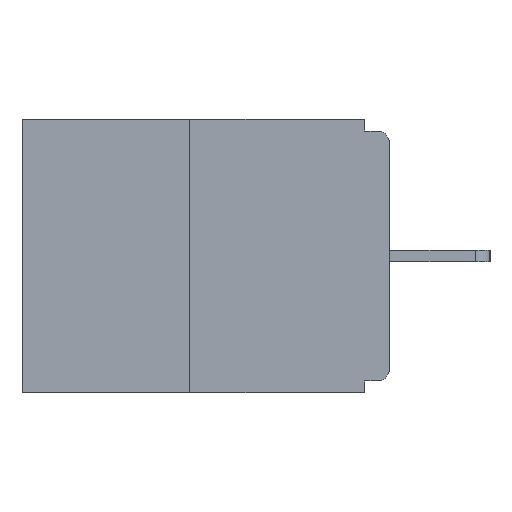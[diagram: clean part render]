
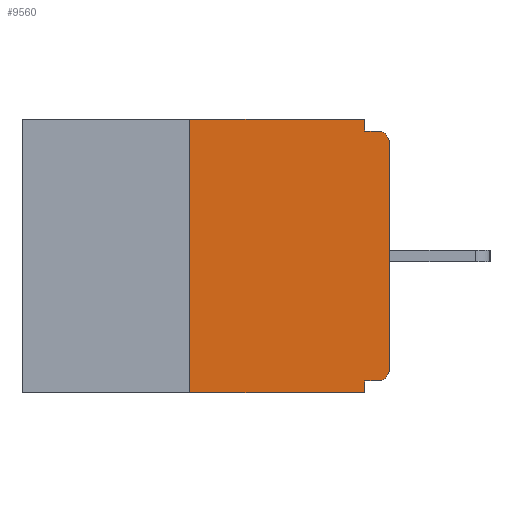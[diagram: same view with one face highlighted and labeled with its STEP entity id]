
A CAD part, left-side view. The second image highlights one B-rep face of the part: STEP entity #9560.
In plain terms, the highlighted planar face has unit normal (-1, 0, 0).
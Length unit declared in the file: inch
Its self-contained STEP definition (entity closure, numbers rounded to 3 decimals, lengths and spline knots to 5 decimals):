
#99 = DIRECTION ( 'NONE',  ( 0., 0., 1. ) ) ;
#216 = ORIENTED_EDGE ( 'NONE', *, *, #5805, .F. ) ;
#753 = CARTESIAN_POINT ( 'NONE',  ( 0., 0.015, -0.328 ) ) ;
#810 = CARTESIAN_POINT ( 'NONE',  ( 0., 0.031, -0.328 ) ) ;
#871 = CARTESIAN_POINT ( 'NONE',  ( 0., 0.031, -0.015 ) ) ;
#1136 = VERTEX_POINT ( 'NONE', #871 ) ;
#1218 = LINE ( 'NONE', #10630, #3460 ) ;
#1287 = AXIS2_PLACEMENT_3D ( 'NONE', #2479, #9513, #3595 ) ;
#1617 = CARTESIAN_POINT ( 'NONE',  ( 0., 0.25, 0. ) ) ;
#1647 = EDGE_CURVE ( 'NONE', #8354, #12426, #13458, .T. ) ;
#1669 = ORIENTED_EDGE ( 'NONE', *, *, #9038, .F. ) ;
#1750 = EDGE_CURVE ( 'NONE', #1136, #12426, #6166, .T. ) ;
#1998 = VERTEX_POINT ( 'NONE', #753 ) ;
#2083 = ORIENTED_EDGE ( 'NONE', *, *, #9638, .F. ) ;
#2479 = CARTESIAN_POINT ( 'NONE',  ( 0., 0.015, -0.313 ) ) ;
#2496 = AXIS2_PLACEMENT_3D ( 'NONE', #7346, #9879, #7579 ) ;
#2565 = VECTOR ( 'NONE', #99, 39.37008 ) ;
#2848 = EDGE_CURVE ( 'NONE', #10199, #1136, #1218, .T. ) ;
#2975 = VERTEX_POINT ( 'NONE', #11094 ) ;
#3161 = CARTESIAN_POINT ( 'NONE',  ( 0., 0.031, 0. ) ) ;
#3400 = CARTESIAN_POINT ( 'NONE',  ( 0., 0., -0.328 ) ) ;
#3460 = VECTOR ( 'NONE', #14411, 39.37008 ) ;
#3528 = DIRECTION ( 'NONE',  ( 0., -1., 0. ) ) ;
#3595 = DIRECTION ( 'NONE',  ( 0., 0., -1. ) ) ;
#4274 = VECTOR ( 'NONE', #14276, 39.37008 ) ;
#4645 = CARTESIAN_POINT ( 'NONE',  ( 0., 0., 0. ) ) ;
#4684 = DIRECTION ( 'NONE',  ( -1., 0., 0. ) ) ;
#4777 = VERTEX_POINT ( 'NONE', #6903 ) ;
#4787 = VERTEX_POINT ( 'NONE', #810 ) ;
#5148 = FACE_OUTER_BOUND ( 'NONE', #13052, .T. ) ;
#5202 = ORIENTED_EDGE ( 'NONE', *, *, #1750, .F. ) ;
#5406 = DIRECTION ( 'NONE',  ( 0., 0., -1. ) ) ;
#5527 = CARTESIAN_POINT ( 'NONE',  ( 0., 0.25, -0.343 ) ) ;
#5589 = VERTEX_POINT ( 'NONE', #5527 ) ;
#5799 = LINE ( 'NONE', #7056, #11694 ) ;
#5805 = EDGE_CURVE ( 'NONE', #1998, #4787, #15034, .T. ) ;
#6166 = LINE ( 'NONE', #10734, #4274 ) ;
#6281 = DIRECTION ( 'NONE',  ( 0., -1., 0. ) ) ;
#6903 = CARTESIAN_POINT ( 'NONE',  ( 0., 0.25, 0. ) ) ;
#7026 = CIRCLE ( 'NONE', #1287, 0.015 ) ;
#7030 = CARTESIAN_POINT ( 'NONE',  ( 0., 0.015, -0.03 ) ) ;
#7056 = CARTESIAN_POINT ( 'NONE',  ( 0., 0.46, 0. ) ) ;
#7135 = VECTOR ( 'NONE', #5406, 39.37008 ) ;
#7346 = CARTESIAN_POINT ( 'NONE',  ( 0., 0.46, 0. ) ) ;
#7377 = EDGE_CURVE ( 'NONE', #5589, #2975, #14381, .T. ) ;
#7572 = EDGE_CURVE ( 'NONE', #4787, #2975, #10304, .T. ) ;
#7579 = DIRECTION ( 'NONE',  ( 0., 0., -1. ) ) ;
#7812 = DIRECTION ( 'NONE',  ( 0., 0., 1. ) ) ;
#7888 = ORIENTED_EDGE ( 'NONE', *, *, #12961, .T. ) ;
#8354 = VERTEX_POINT ( 'NONE', #15089 ) ;
#8446 = VERTEX_POINT ( 'NONE', #14858 ) ;
#8518 = CARTESIAN_POINT ( 'NONE',  ( 0., 0.46, -0.343 ) ) ;
#9017 = VECTOR ( 'NONE', #6281, 39.37008 ) ;
#9038 = EDGE_CURVE ( 'NONE', #4777, #10199, #5799, .T. ) ;
#9131 = CARTESIAN_POINT ( 'NONE',  ( 0., 0.031, -0.343 ) ) ;
#9264 = VECTOR ( 'NONE', #15105, 39.37008 ) ;
#9513 = DIRECTION ( 'NONE',  ( -1., 0., 0. ) ) ;
#9560 = ADVANCED_FACE ( 'NONE', ( #5148 ), #10733, .F. ) ;
#9638 = EDGE_CURVE ( 'NONE', #5589, #4777, #15038, .T. ) ;
#9769 = ORIENTED_EDGE ( 'NONE', *, *, #2848, .F. ) ;
#9879 = DIRECTION ( 'NONE',  ( 1., 0., 0. ) ) ;
#10173 = CARTESIAN_POINT ( 'NONE',  ( 0., 0.015, -0.015 ) ) ;
#10199 = VERTEX_POINT ( 'NONE', #3161 ) ;
#10304 = LINE ( 'NONE', #9131, #7135 ) ;
#10630 = CARTESIAN_POINT ( 'NONE',  ( 0., 0.031, 0. ) ) ;
#10733 = PLANE ( 'NONE',  #2496 ) ;
#10734 = CARTESIAN_POINT ( 'NONE',  ( 0., 0., -0.015 ) ) ;
#11094 = CARTESIAN_POINT ( 'NONE',  ( 0., 0.031, -0.343 ) ) ;
#11532 = DIRECTION ( 'NONE',  ( 0., 0., -1. ) ) ;
#11694 = VECTOR ( 'NONE', #3528, 39.37008 ) ;
#11828 = EDGE_CURVE ( 'NONE', #1998, #8446, #7026, .T. ) ;
#12426 = VERTEX_POINT ( 'NONE', #10173 ) ;
#12961 = EDGE_CURVE ( 'NONE', #8446, #8354, #13193, .T. ) ;
#13052 = EDGE_LOOP ( 'NONE', ( #1669, #2083, #14701, #14960, #216, #13875, #7888, #15066, #5202, #9769 ) ) ;
#13193 = LINE ( 'NONE', #4645, #2565 ) ;
#13458 = CIRCLE ( 'NONE', #14715, 0.015 ) ;
#13875 = ORIENTED_EDGE ( 'NONE', *, *, #11828, .T. ) ;
#14276 = DIRECTION ( 'NONE',  ( 0., -1., 0. ) ) ;
#14381 = LINE ( 'NONE', #8518, #9017 ) ;
#14411 = DIRECTION ( 'NONE',  ( 0., 0., -1. ) ) ;
#14701 = ORIENTED_EDGE ( 'NONE', *, *, #7377, .T. ) ;
#14715 = AXIS2_PLACEMENT_3D ( 'NONE', #7030, #4684, #11532 ) ;
#14717 = VECTOR ( 'NONE', #7812, 39.37008 ) ;
#14858 = CARTESIAN_POINT ( 'NONE',  ( 0., 0., -0.313 ) ) ;
#14960 = ORIENTED_EDGE ( 'NONE', *, *, #7572, .F. ) ;
#15034 = LINE ( 'NONE', #3400, #9264 ) ;
#15038 = LINE ( 'NONE', #1617, #14717 ) ;
#15066 = ORIENTED_EDGE ( 'NONE', *, *, #1647, .T. ) ;
#15089 = CARTESIAN_POINT ( 'NONE',  ( 0., 0., -0.03 ) ) ;
#15105 = DIRECTION ( 'NONE',  ( 0., 1., 0. ) ) ;
